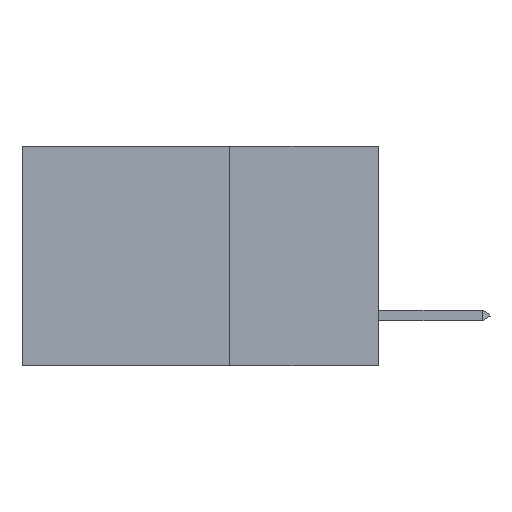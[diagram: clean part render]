
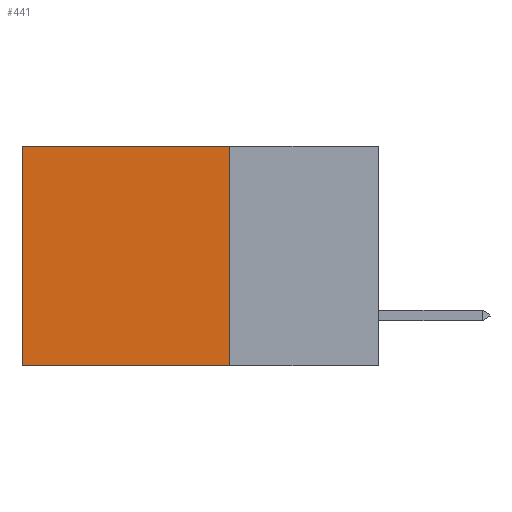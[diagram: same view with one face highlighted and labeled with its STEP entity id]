
A CAD part, left-side view. The second image highlights one B-rep face of the part: STEP entity #441.
In plain terms, the highlighted planar face has unit normal (-1, 0, 0).
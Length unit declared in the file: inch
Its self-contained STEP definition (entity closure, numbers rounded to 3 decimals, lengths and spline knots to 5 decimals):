
#207 = EDGE_CURVE ( 'NONE', #1093, #9288, #4691, .T. ) ;
#311 = VERTEX_POINT ( 'NONE', #3323 ) ;
#441 = ADVANCED_FACE ( 'NONE', ( #1568 ), #1108, .F. ) ;
#608 = CARTESIAN_POINT ( 'NONE',  ( 0.298, 0.6, 0. ) ) ;
#1093 = VERTEX_POINT ( 'NONE', #10571 ) ;
#1108 = PLANE ( 'NONE',  #6238 ) ;
#1568 = FACE_OUTER_BOUND ( 'NONE', #8719, .T. ) ;
#1594 = CARTESIAN_POINT ( 'NONE',  ( 0.298, 0.6, 0. ) ) ;
#1729 = CARTESIAN_POINT ( 'NONE',  ( 0.298, 0.25, 0. ) ) ;
#2254 = DIRECTION ( 'NONE',  ( 0., 0., -1. ) ) ;
#2647 = EDGE_CURVE ( 'NONE', #1093, #311, #12674, .T. ) ;
#3323 = CARTESIAN_POINT ( 'NONE',  ( 0.298, 0.25, -0.37 ) ) ;
#3808 = ORIENTED_EDGE ( 'NONE', *, *, #9320, .T. ) ;
#4387 = VERTEX_POINT ( 'NONE', #8293 ) ;
#4691 = LINE ( 'NONE', #10097, #10247 ) ;
#5052 = ORIENTED_EDGE ( 'NONE', *, *, #207, .T. ) ;
#5221 = ORIENTED_EDGE ( 'NONE', *, *, #6849, .F. ) ;
#5605 = ORIENTED_EDGE ( 'NONE', *, *, #2647, .F. ) ;
#6217 = DIRECTION ( 'NONE',  ( 0., 1., 0. ) ) ;
#6238 = AXIS2_PLACEMENT_3D ( 'NONE', #8057, #11204, #2254 ) ;
#6849 = EDGE_CURVE ( 'NONE', #311, #4387, #8736, .T. ) ;
#7326 = VECTOR ( 'NONE', #8071, 39.37008 ) ;
#7560 = DIRECTION ( 'NONE',  ( 0., 0., -1. ) ) ;
#7989 = CARTESIAN_POINT ( 'NONE',  ( 0.298, 0.25, -0.37 ) ) ;
#8057 = CARTESIAN_POINT ( 'NONE',  ( 0.298, 0.25, 0. ) ) ;
#8071 = DIRECTION ( 'NONE',  ( 0., 1., 0. ) ) ;
#8293 = CARTESIAN_POINT ( 'NONE',  ( 0.298, 0.6, -0.37 ) ) ;
#8359 = VECTOR ( 'NONE', #7560, 39.37008 ) ;
#8719 = EDGE_LOOP ( 'NONE', ( #3808, #5221, #5605, #5052 ) ) ;
#8736 = LINE ( 'NONE', #7989, #7326 ) ;
#9288 = VERTEX_POINT ( 'NONE', #1594 ) ;
#9320 = EDGE_CURVE ( 'NONE', #9288, #4387, #10054, .T. ) ;
#10054 = LINE ( 'NONE', #608, #8359 ) ;
#10097 = CARTESIAN_POINT ( 'NONE',  ( 0.298, 0.25, 0. ) ) ;
#10171 = VECTOR ( 'NONE', #12582, 39.37008 ) ;
#10247 = VECTOR ( 'NONE', #6217, 39.37008 ) ;
#10571 = CARTESIAN_POINT ( 'NONE',  ( 0.298, 0.25, 0. ) ) ;
#11204 = DIRECTION ( 'NONE',  ( 1., 0., 0. ) ) ;
#12582 = DIRECTION ( 'NONE',  ( 0., 0., -1. ) ) ;
#12674 = LINE ( 'NONE', #1729, #10171 ) ;
